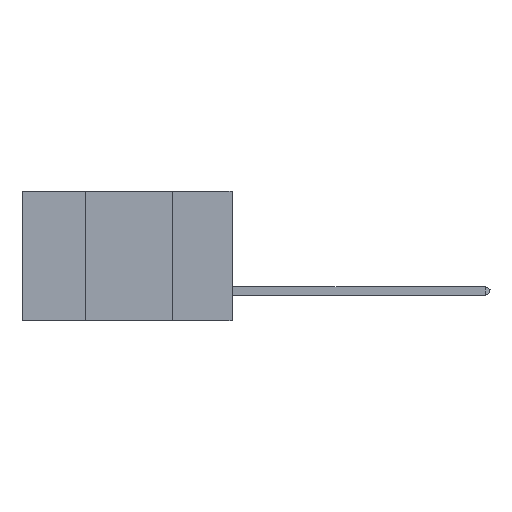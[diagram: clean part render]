
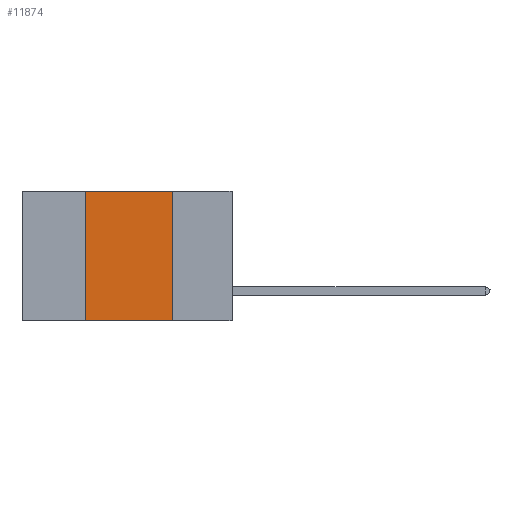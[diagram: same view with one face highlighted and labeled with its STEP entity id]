
A CAD part, left-side view. The second image highlights one B-rep face of the part: STEP entity #11874.
In plain terms, the highlighted planar face has unit normal (-1, 0, 0).
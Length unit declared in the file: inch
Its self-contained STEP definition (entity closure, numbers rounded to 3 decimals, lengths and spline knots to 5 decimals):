
#1106 = EDGE_CURVE ( 'NONE', #23261, #1868, #18813, .T. ) ;
#1152 = CARTESIAN_POINT ( 'NONE',  ( 0., 0.6, -0.37 ) ) ;
#1291 = DIRECTION ( 'NONE',  ( 1., 0., 0. ) ) ;
#1868 = VERTEX_POINT ( 'NONE', #8034 ) ;
#1892 = VECTOR ( 'NONE', #15299, 39.37008 ) ;
#2767 = EDGE_LOOP ( 'NONE', ( #6413, #6691, #8648, #16747 ) ) ;
#3227 = CARTESIAN_POINT ( 'NONE',  ( 0., 0.42, -0.37 ) ) ;
#3355 = DIRECTION ( 'NONE',  ( 0., 0., -1. ) ) ;
#3512 = EDGE_CURVE ( 'NONE', #1868, #10845, #15467, .T. ) ;
#4273 = CARTESIAN_POINT ( 'NONE',  ( 0., 0.42, 0. ) ) ;
#6413 = ORIENTED_EDGE ( 'NONE', *, *, #18269, .F. ) ;
#6691 = ORIENTED_EDGE ( 'NONE', *, *, #3512, .F. ) ;
#8034 = CARTESIAN_POINT ( 'NONE',  ( 0., 0.42, 0. ) ) ;
#8602 = LINE ( 'NONE', #16201, #10025 ) ;
#8648 = ORIENTED_EDGE ( 'NONE', *, *, #1106, .F. ) ;
#9057 = VECTOR ( 'NONE', #16068, 39.37008 ) ;
#10025 = VECTOR ( 'NONE', #3355, 39.37008 ) ;
#10298 = CARTESIAN_POINT ( 'NONE',  ( 0., 0.17, 0. ) ) ;
#10791 = DIRECTION ( 'NONE',  ( 0., 0., -1. ) ) ;
#10845 = VERTEX_POINT ( 'NONE', #10298 ) ;
#11677 = VECTOR ( 'NONE', #21036, 39.37008 ) ;
#11874 = ADVANCED_FACE ( 'NONE', ( #16685 ), #15715, .F. ) ;
#12785 = CARTESIAN_POINT ( 'NONE',  ( 0., 0.6, 0. ) ) ;
#13016 = EDGE_CURVE ( 'NONE', #23261, #14977, #17824, .T. ) ;
#14977 = VERTEX_POINT ( 'NONE', #23605 ) ;
#15299 = DIRECTION ( 'NONE',  ( 0., 0., 1. ) ) ;
#15467 = LINE ( 'NONE', #12785, #11677 ) ;
#15715 = PLANE ( 'NONE',  #16841 ) ;
#16068 = DIRECTION ( 'NONE',  ( 0., -1., 0. ) ) ;
#16201 = CARTESIAN_POINT ( 'NONE',  ( 0., 0.17, 0. ) ) ;
#16685 = FACE_OUTER_BOUND ( 'NONE', #2767, .T. ) ;
#16747 = ORIENTED_EDGE ( 'NONE', *, *, #13016, .T. ) ;
#16841 = AXIS2_PLACEMENT_3D ( 'NONE', #17591, #1291, #10791 ) ;
#17591 = CARTESIAN_POINT ( 'NONE',  ( 0., 0.6, 0. ) ) ;
#17824 = LINE ( 'NONE', #1152, #9057 ) ;
#18269 = EDGE_CURVE ( 'NONE', #10845, #14977, #8602, .T. ) ;
#18813 = LINE ( 'NONE', #4273, #1892 ) ;
#21036 = DIRECTION ( 'NONE',  ( 0., -1., 0. ) ) ;
#23261 = VERTEX_POINT ( 'NONE', #3227 ) ;
#23605 = CARTESIAN_POINT ( 'NONE',  ( 0., 0.17, -0.37 ) ) ;
